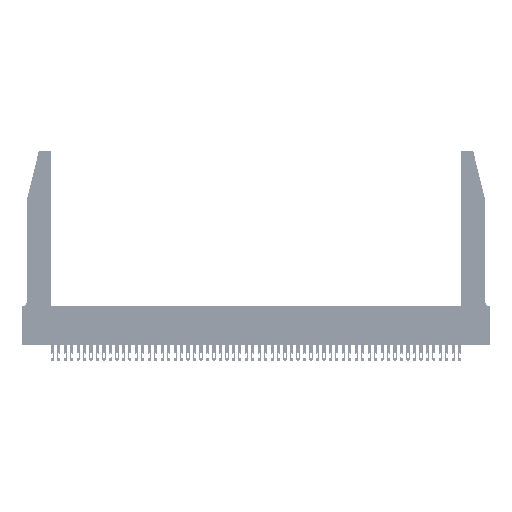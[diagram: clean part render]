
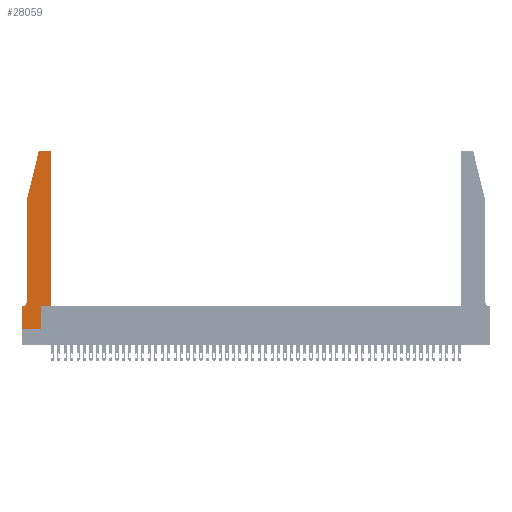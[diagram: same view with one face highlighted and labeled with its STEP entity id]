
A CAD part, top view. The second image highlights one B-rep face of the part: STEP entity #28059.
In plain terms, the highlighted planar face has unit normal (0, 0, 1).
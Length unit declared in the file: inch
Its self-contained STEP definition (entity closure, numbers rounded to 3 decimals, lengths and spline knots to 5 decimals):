
#631 = VECTOR ( 'NONE', #915, 39.37008 ) ;
#915 = DIRECTION ( 'NONE',  ( -1., 0., 0. ) ) ;
#1359 = CARTESIAN_POINT ( 'NONE',  ( 0.0055, 0.35, 0.37 ) ) ;
#1388 = EDGE_CURVE ( 'NONE', #26448, #3122, #31455, .T. ) ;
#1684 = CARTESIAN_POINT ( 'NONE',  ( 0., 0.35, 0.37 ) ) ;
#1687 = VERTEX_POINT ( 'NONE', #1684 ) ;
#1848 = VECTOR ( 'NONE', #21329, 39.37008 ) ;
#2250 = CARTESIAN_POINT ( 'NONE',  ( 0.2865, 0., 0.37 ) ) ;
#3122 = VERTEX_POINT ( 'NONE', #47793 ) ;
#3802 = EDGE_CURVE ( 'NONE', #37878, #37928, #32482, .T. ) ;
#4156 = ORIENTED_EDGE ( 'NONE', *, *, #48045, .T. ) ;
#4191 = CARTESIAN_POINT ( 'NONE',  ( 0.4205, 2.72, 0.37 ) ) ;
#4271 = DIRECTION ( 'NONE',  ( -1., 0., 0. ) ) ;
#4733 = LINE ( 'NONE', #36566, #48656 ) ;
#5308 = CIRCLE ( 'NONE', #17803, 0.07 ) ;
#6887 = ORIENTED_EDGE ( 'NONE', *, *, #48832, .T. ) ;
#7354 = VECTOR ( 'NONE', #28354, 39.37008 ) ;
#7796 = VERTEX_POINT ( 'NONE', #1359 ) ;
#8795 = ORIENTED_EDGE ( 'NONE', *, *, #1388, .T. ) ;
#9016 = CARTESIAN_POINT ( 'NONE',  ( 0.0755, 0.35, 0.37 ) ) ;
#9551 = ORIENTED_EDGE ( 'NONE', *, *, #38225, .T. ) ;
#10023 = VERTEX_POINT ( 'NONE', #36080 ) ;
#10208 = CIRCLE ( 'NONE', #34965, 0.03 ) ;
#10313 = VERTEX_POINT ( 'NONE', #14112 ) ;
#10686 = EDGE_LOOP ( 'NONE', ( #29791, #51642, #9551, #14414, #48648, #20040, #6887, #15216, #33539, #8795, #4156, #50109 ) ) ;
#10829 = EDGE_CURVE ( 'NONE', #19889, #25759, #10208, .T. ) ;
#10860 = VECTOR ( 'NONE', #35235, 39.37008 ) ;
#11136 = PLANE ( 'NONE',  #16960 ) ;
#13195 = VECTOR ( 'NONE', #34639, 39.37008 ) ;
#13693 = VERTEX_POINT ( 'NONE', #2250 ) ;
#13777 = CARTESIAN_POINT ( 'NONE',  ( 0.2865, 0.35, 0.37 ) ) ;
#13938 = CARTESIAN_POINT ( 'NONE',  ( 0.284, 2.72, 0.37 ) ) ;
#14112 = CARTESIAN_POINT ( 'NONE',  ( 0.284, 2.75, 0.37 ) ) ;
#14414 = ORIENTED_EDGE ( 'NONE', *, *, #3802, .T. ) ;
#14943 = VERTEX_POINT ( 'NONE', #36341 ) ;
#15216 = ORIENTED_EDGE ( 'NONE', *, *, #47054, .T. ) ;
#15301 = LINE ( 'NONE', #43288, #10860 ) ;
#16960 = AXIS2_PLACEMENT_3D ( 'NONE', #43225, #19231, #47237 ) ;
#17803 = AXIS2_PLACEMENT_3D ( 'NONE', #48452, #36390, #4271 ) ;
#19231 = DIRECTION ( 'NONE',  ( 0., 0., 1. ) ) ;
#19572 = DIRECTION ( 'NONE',  ( 0., -1., 0. ) ) ;
#19889 = VERTEX_POINT ( 'NONE', #30806 ) ;
#19922 = CARTESIAN_POINT ( 'NONE',  ( 0., 0., 0.37 ) ) ;
#20040 = ORIENTED_EDGE ( 'NONE', *, *, #39131, .T. ) ;
#21045 = DIRECTION ( 'NONE',  ( 0., 0., 1. ) ) ;
#21329 = DIRECTION ( 'NONE',  ( 0., 1., 0. ) ) ;
#22178 = DIRECTION ( 'NONE',  ( 1., 0., 0. ) ) ;
#22201 = CARTESIAN_POINT ( 'NONE',  ( 0.0755, 2., 0.37 ) ) ;
#22446 = EDGE_CURVE ( 'NONE', #37928, #7796, #5308, .T. ) ;
#23891 = CIRCLE ( 'NONE', #29932, 0.03 ) ;
#25575 = CARTESIAN_POINT ( 'NONE',  ( 0.0755, 2., 0.37 ) ) ;
#25759 = VERTEX_POINT ( 'NONE', #49989 ) ;
#26395 = VECTOR ( 'NONE', #31585, 39.37008 ) ;
#26448 = VERTEX_POINT ( 'NONE', #37775 ) ;
#27865 = CARTESIAN_POINT ( 'NONE',  ( 0.4505, 0.35, 0.37 ) ) ;
#28059 = ADVANCED_FACE ( 'NONE', ( #33383 ), #11136, .T. ) ;
#28149 = DIRECTION ( 'NONE',  ( -0.239, -0.971, 0. ) ) ;
#28297 = DIRECTION ( 'NONE',  ( 1., 0., 0. ) ) ;
#28354 = DIRECTION ( 'NONE',  ( 0., -1., 0. ) ) ;
#29791 = ORIENTED_EDGE ( 'NONE', *, *, #50627, .T. ) ;
#29932 = AXIS2_PLACEMENT_3D ( 'NONE', #13938, #38468, #22178 ) ;
#30806 = CARTESIAN_POINT ( 'NONE',  ( 0.4505, 2.72, 0.37 ) ) ;
#31455 = LINE ( 'NONE', #27865, #26395 ) ;
#31585 = DIRECTION ( 'NONE',  ( 1., 0., 0. ) ) ;
#32482 = LINE ( 'NONE', #22201, #7354 ) ;
#33383 = FACE_OUTER_BOUND ( 'NONE', #10686, .T. ) ;
#33539 = ORIENTED_EDGE ( 'NONE', *, *, #35809, .T. ) ;
#33817 = CARTESIAN_POINT ( 'NONE',  ( 0.0755, 0.42, 0.37 ) ) ;
#34639 = DIRECTION ( 'NONE',  ( -1., 0., 0. ) ) ;
#34965 = AXIS2_PLACEMENT_3D ( 'NONE', #4191, #21045, #39793 ) ;
#35235 = DIRECTION ( 'NONE',  ( 0., 1., 0. ) ) ;
#35809 = EDGE_CURVE ( 'NONE', #13693, #26448, #49561, .T. ) ;
#36080 = CARTESIAN_POINT ( 'NONE',  ( 0.25487, 2.72718, 0.37 ) ) ;
#36341 = CARTESIAN_POINT ( 'NONE',  ( 0., 0., 0.37 ) ) ;
#36390 = DIRECTION ( 'NONE',  ( 0., 0., -1. ) ) ;
#36566 = CARTESIAN_POINT ( 'NONE',  ( 0., 0., 0.37 ) ) ;
#36813 = EDGE_CURVE ( 'NONE', #10313, #10023, #23891, .T. ) ;
#37775 = CARTESIAN_POINT ( 'NONE',  ( 0.2865, 0.35, 0.37 ) ) ;
#37878 = VERTEX_POINT ( 'NONE', #25575 ) ;
#37928 = VERTEX_POINT ( 'NONE', #33817 ) ;
#38225 = EDGE_CURVE ( 'NONE', #10023, #37878, #43373, .T. ) ;
#38337 = VECTOR ( 'NONE', #28149, 39.37008 ) ;
#38388 = LINE ( 'NONE', #19922, #44031 ) ;
#38468 = DIRECTION ( 'NONE',  ( 0., 0., 1. ) ) ;
#39131 = EDGE_CURVE ( 'NONE', #7796, #1687, #51466, .T. ) ;
#39393 = CARTESIAN_POINT ( 'NONE',  ( 0.0755, 2., 0.37 ) ) ;
#39793 = DIRECTION ( 'NONE',  ( 1., 0., 0. ) ) ;
#43225 = CARTESIAN_POINT ( 'NONE',  ( 0., 0.35, 0.37 ) ) ;
#43288 = CARTESIAN_POINT ( 'NONE',  ( 0.4505, 0.35, 0.37 ) ) ;
#43373 = LINE ( 'NONE', #39393, #38337 ) ;
#44031 = VECTOR ( 'NONE', #19572, 39.37008 ) ;
#45181 = LINE ( 'NONE', #50400, #13195 ) ;
#47054 = EDGE_CURVE ( 'NONE', #14943, #13693, #4733, .T. ) ;
#47237 = DIRECTION ( 'NONE',  ( 1., 0., 0. ) ) ;
#47793 = CARTESIAN_POINT ( 'NONE',  ( 0.4505, 0.35, 0.37 ) ) ;
#48045 = EDGE_CURVE ( 'NONE', #3122, #19889, #15301, .T. ) ;
#48452 = CARTESIAN_POINT ( 'NONE',  ( 0.0055, 0.42, 0.37 ) ) ;
#48648 = ORIENTED_EDGE ( 'NONE', *, *, #22446, .T. ) ;
#48656 = VECTOR ( 'NONE', #28297, 39.37008 ) ;
#48832 = EDGE_CURVE ( 'NONE', #1687, #14943, #38388, .T. ) ;
#49561 = LINE ( 'NONE', #13777, #1848 ) ;
#49989 = CARTESIAN_POINT ( 'NONE',  ( 0.4205, 2.75, 0.37 ) ) ;
#50109 = ORIENTED_EDGE ( 'NONE', *, *, #10829, .T. ) ;
#50400 = CARTESIAN_POINT ( 'NONE',  ( 0.2605, 2.75, 0.37 ) ) ;
#50627 = EDGE_CURVE ( 'NONE', #25759, #10313, #45181, .T. ) ;
#51466 = LINE ( 'NONE', #9016, #631 ) ;
#51642 = ORIENTED_EDGE ( 'NONE', *, *, #36813, .T. ) ;
